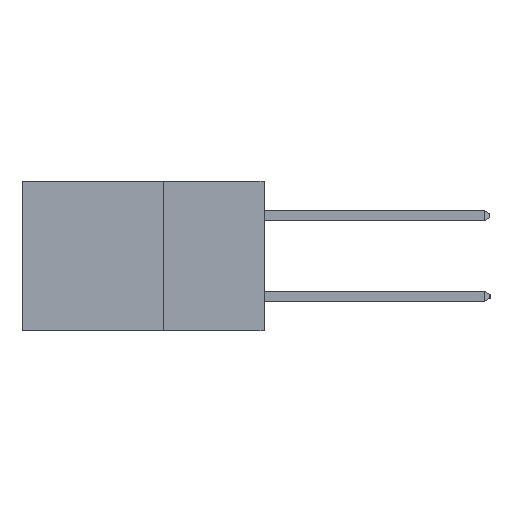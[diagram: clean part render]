
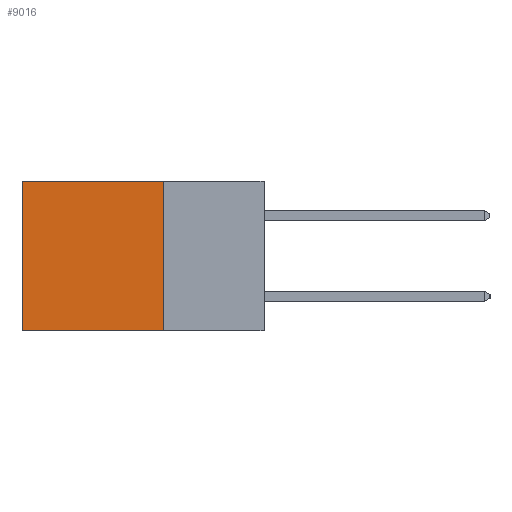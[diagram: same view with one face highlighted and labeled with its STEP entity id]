
A CAD part, left-side view. The second image highlights one B-rep face of the part: STEP entity #9016.
In plain terms, the highlighted planar face has unit normal (-1, 0, 0).
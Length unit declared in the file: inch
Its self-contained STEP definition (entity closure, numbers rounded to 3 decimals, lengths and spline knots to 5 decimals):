
#752 = CARTESIAN_POINT ( 'NONE',  ( 0.2615, 0.6, 0. ) ) ;
#1050 = ORIENTED_EDGE ( 'NONE', *, *, #2993, .T. ) ;
#2060 = EDGE_CURVE ( 'NONE', #4954, #6340, #8755, .T. ) ;
#2641 = CARTESIAN_POINT ( 'NONE',  ( 0.2615, 0.6, -0.37 ) ) ;
#2982 = CARTESIAN_POINT ( 'NONE',  ( 0.2615, 0.25, -0.37 ) ) ;
#2993 = EDGE_CURVE ( 'NONE', #5758, #4954, #7083, .T. ) ;
#2998 = PLANE ( 'NONE',  #8929 ) ;
#3054 = DIRECTION ( 'NONE',  ( 0., 0., -1. ) ) ;
#3115 = CARTESIAN_POINT ( 'NONE',  ( 0.2615, 0.25, -0.37 ) ) ;
#3304 = VECTOR ( 'NONE', #8906, 39.37008 ) ;
#3332 = DIRECTION ( 'NONE',  ( 0., 0., -1. ) ) ;
#3481 = VECTOR ( 'NONE', #8484, 39.37008 ) ;
#3570 = EDGE_CURVE ( 'NONE', #5758, #5481, #7649, .T. ) ;
#4039 = CARTESIAN_POINT ( 'NONE',  ( 0.2615, 0.25, 0. ) ) ;
#4189 = CARTESIAN_POINT ( 'NONE',  ( 0.2615, 0.6, -0.37 ) ) ;
#4219 = CARTESIAN_POINT ( 'NONE',  ( 0.2615, 0.25, 0. ) ) ;
#4525 = DIRECTION ( 'NONE',  ( 0., 0., -1. ) ) ;
#4629 = ORIENTED_EDGE ( 'NONE', *, *, #2060, .T. ) ;
#4954 = VERTEX_POINT ( 'NONE', #752 ) ;
#5481 = VERTEX_POINT ( 'NONE', #6271 ) ;
#5543 = LINE ( 'NONE', #3115, #3481 ) ;
#5686 = VECTOR ( 'NONE', #3332, 39.37008 ) ;
#5758 = VERTEX_POINT ( 'NONE', #4219 ) ;
#6219 = EDGE_CURVE ( 'NONE', #5481, #6340, #5543, .T. ) ;
#6271 = CARTESIAN_POINT ( 'NONE',  ( 0.2615, 0.25, -0.37 ) ) ;
#6340 = VERTEX_POINT ( 'NONE', #4189 ) ;
#6824 = ORIENTED_EDGE ( 'NONE', *, *, #3570, .F. ) ;
#6880 = VECTOR ( 'NONE', #3054, 39.37008 ) ;
#7083 = LINE ( 'NONE', #4039, #3304 ) ;
#7649 = LINE ( 'NONE', #2982, #5686 ) ;
#8187 = CARTESIAN_POINT ( 'NONE',  ( 0.2615, 0.25, -0.37 ) ) ;
#8342 = FACE_OUTER_BOUND ( 'NONE', #8584, .T. ) ;
#8484 = DIRECTION ( 'NONE',  ( 0., 1., 0. ) ) ;
#8508 = ORIENTED_EDGE ( 'NONE', *, *, #6219, .F. ) ;
#8584 = EDGE_LOOP ( 'NONE', ( #4629, #8508, #6824, #1050 ) ) ;
#8755 = LINE ( 'NONE', #2641, #6880 ) ;
#8882 = DIRECTION ( 'NONE',  ( 1., 0., 0. ) ) ;
#8906 = DIRECTION ( 'NONE',  ( 0., 1., 0. ) ) ;
#8929 = AXIS2_PLACEMENT_3D ( 'NONE', #8187, #8882, #4525 ) ;
#9016 = ADVANCED_FACE ( 'NONE', ( #8342 ), #2998, .F. ) ;
